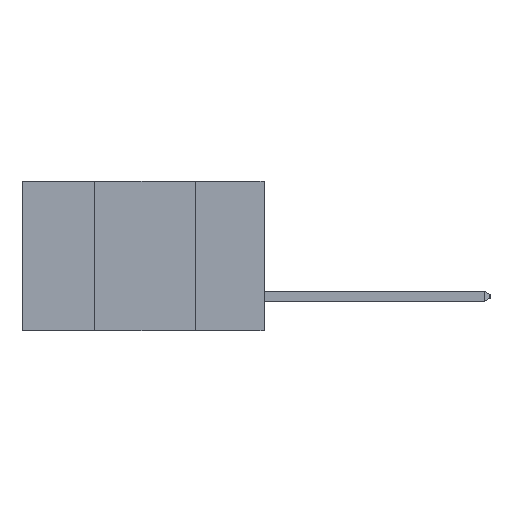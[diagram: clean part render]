
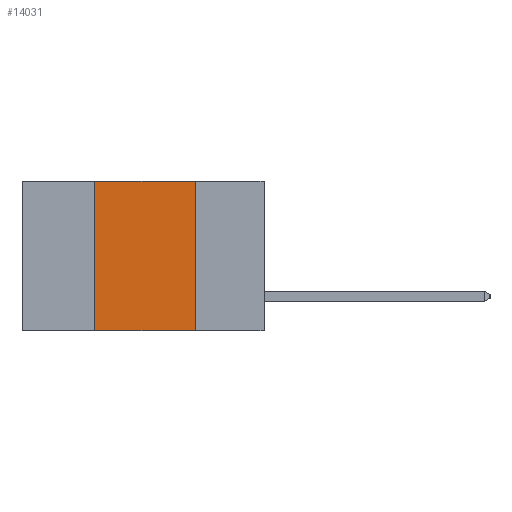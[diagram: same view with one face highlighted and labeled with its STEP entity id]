
A CAD part, left-side view. The second image highlights one B-rep face of the part: STEP entity #14031.
In plain terms, the highlighted planar face has unit normal (-1, 0, 0).
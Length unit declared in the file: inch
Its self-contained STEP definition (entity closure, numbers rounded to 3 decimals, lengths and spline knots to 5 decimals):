
#210 = VECTOR ( 'NONE', #11592, 39.37008 ) ;
#651 = VECTOR ( 'NONE', #5109, 39.37008 ) ;
#1062 = EDGE_CURVE ( 'NONE', #16405, #11317, #6463, .T. ) ;
#1281 = DIRECTION ( 'NONE',  ( 0., 0., -1. ) ) ;
#1530 = ORIENTED_EDGE ( 'NONE', *, *, #3534, .F. ) ;
#1535 = DIRECTION ( 'NONE',  ( 0., -1., 0. ) ) ;
#1624 = CARTESIAN_POINT ( 'NONE',  ( 0., 0.6, 0. ) ) ;
#2390 = EDGE_CURVE ( 'NONE', #15634, #4040, #4115, .T. ) ;
#2684 = EDGE_CURVE ( 'NONE', #16405, #15634, #14697, .T. ) ;
#3534 = EDGE_CURVE ( 'NONE', #4040, #11317, #8630, .T. ) ;
#3755 = EDGE_LOOP ( 'NONE', ( #1530, #7296, #13610, #5106 ) ) ;
#4040 = VERTEX_POINT ( 'NONE', #7984 ) ;
#4115 = LINE ( 'NONE', #1624, #210 ) ;
#5106 = ORIENTED_EDGE ( 'NONE', *, *, #1062, .T. ) ;
#5109 = DIRECTION ( 'NONE',  ( 0., 0., -1. ) ) ;
#5536 = PLANE ( 'NONE',  #12888 ) ;
#5735 = CARTESIAN_POINT ( 'NONE',  ( 0., 0.42, -0.37 ) ) ;
#6463 = LINE ( 'NONE', #9420, #17067 ) ;
#6487 = CARTESIAN_POINT ( 'NONE',  ( 0., 0.42, 0. ) ) ;
#7296 = ORIENTED_EDGE ( 'NONE', *, *, #2390, .F. ) ;
#7907 = DIRECTION ( 'NONE',  ( 0., 0., 1. ) ) ;
#7984 = CARTESIAN_POINT ( 'NONE',  ( 0., 0.17, 0. ) ) ;
#8630 = LINE ( 'NONE', #17365, #651 ) ;
#9420 = CARTESIAN_POINT ( 'NONE',  ( 0., 0.6, -0.37 ) ) ;
#9616 = CARTESIAN_POINT ( 'NONE',  ( 0., 0.17, -0.37 ) ) ;
#9693 = DIRECTION ( 'NONE',  ( 1., 0., 0. ) ) ;
#11317 = VERTEX_POINT ( 'NONE', #9616 ) ;
#11592 = DIRECTION ( 'NONE',  ( 0., -1., 0. ) ) ;
#12141 = CARTESIAN_POINT ( 'NONE',  ( 0., 0.42, -0.37 ) ) ;
#12888 = AXIS2_PLACEMENT_3D ( 'NONE', #17529, #9693, #1281 ) ;
#13516 = FACE_OUTER_BOUND ( 'NONE', #3755, .T. ) ;
#13610 = ORIENTED_EDGE ( 'NONE', *, *, #2684, .F. ) ;
#14031 = ADVANCED_FACE ( 'NONE', ( #13516 ), #5536, .F. ) ;
#14272 = VECTOR ( 'NONE', #7907, 39.37008 ) ;
#14697 = LINE ( 'NONE', #12141, #14272 ) ;
#15634 = VERTEX_POINT ( 'NONE', #6487 ) ;
#16405 = VERTEX_POINT ( 'NONE', #5735 ) ;
#17067 = VECTOR ( 'NONE', #1535, 39.37008 ) ;
#17365 = CARTESIAN_POINT ( 'NONE',  ( 0., 0.17, -0.37 ) ) ;
#17529 = CARTESIAN_POINT ( 'NONE',  ( 0., 0.6, 0. ) ) ;
